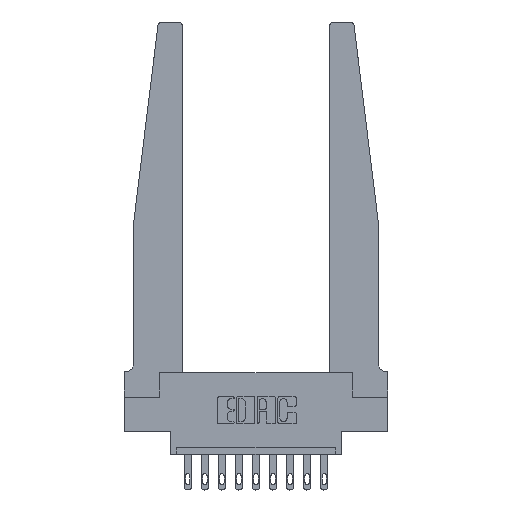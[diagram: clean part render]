
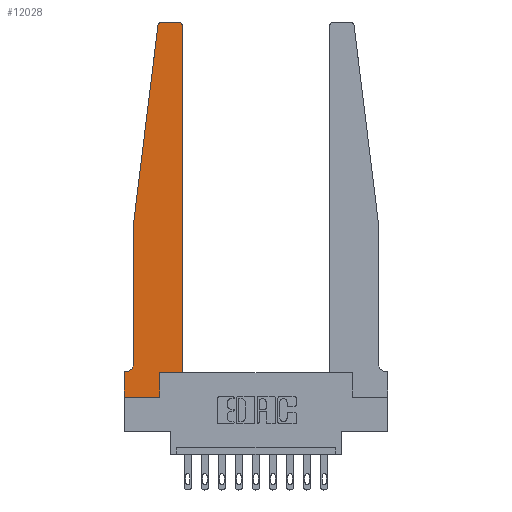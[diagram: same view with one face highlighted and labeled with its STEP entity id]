
A CAD part, top view. The second image highlights one B-rep face of the part: STEP entity #12028.
In plain terms, the highlighted planar face has unit normal (0, 0, 1).
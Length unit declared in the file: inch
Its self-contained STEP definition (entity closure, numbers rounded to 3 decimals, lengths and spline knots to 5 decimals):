
#221 = DIRECTION ( 'NONE',  ( -1., 0., 0. ) ) ;
#763 = ORIENTED_EDGE ( 'NONE', *, *, #5011, .T. ) ;
#813 = EDGE_CURVE ( 'NONE', #10666, #7998, #6678, .T. ) ;
#850 = EDGE_CURVE ( 'NONE', #5270, #13004, #12733, .T. ) ;
#868 = DIRECTION ( 'NONE',  ( 1., 0., 0. ) ) ;
#1016 = DIRECTION ( 'NONE',  ( 0., 0., 1. ) ) ;
#1043 = EDGE_CURVE ( 'NONE', #7309, #5270, #9186, .T. ) ;
#1405 = ORIENTED_EDGE ( 'NONE', *, *, #11373, .T. ) ;
#1758 = ORIENTED_EDGE ( 'NONE', *, *, #3861, .T. ) ;
#1767 = VERTEX_POINT ( 'NONE', #14062 ) ;
#2105 = DIRECTION ( 'NONE',  ( -0.122, -0.992, 0. ) ) ;
#2142 = ORIENTED_EDGE ( 'NONE', *, *, #10994, .T. ) ;
#2347 = CARTESIAN_POINT ( 'NONE',  ( 0., 0.1875, 0.37 ) ) ;
#2426 = ORIENTED_EDGE ( 'NONE', *, *, #3804, .T. ) ;
#2556 = VECTOR ( 'NONE', #3818, 39.37008 ) ;
#2643 = DIRECTION ( 'NONE',  ( -1., 0., 0. ) ) ;
#2780 = LINE ( 'NONE', #10734, #3849 ) ;
#2828 = DIRECTION ( 'NONE',  ( -1., 0., 0. ) ) ;
#2833 = AXIS2_PLACEMENT_3D ( 'NONE', #4006, #8674, #2828 ) ;
#2922 = AXIS2_PLACEMENT_3D ( 'NONE', #9887, #3920, #2981 ) ;
#2929 = VECTOR ( 'NONE', #2105, 39.37008 ) ;
#2981 = DIRECTION ( 'NONE',  ( 1., 0., 0. ) ) ;
#3204 = DIRECTION ( 'NONE',  ( 0., 1., 0. ) ) ;
#3804 = EDGE_CURVE ( 'NONE', #13603, #10203, #5160, .T. ) ;
#3818 = DIRECTION ( 'NONE',  ( 0., -1., 0. ) ) ;
#3849 = VECTOR ( 'NONE', #2643, 39.37008 ) ;
#3861 = EDGE_CURVE ( 'NONE', #6437, #1767, #8073, .T. ) ;
#3920 = DIRECTION ( 'NONE',  ( 0., 0., 1. ) ) ;
#4006 = CARTESIAN_POINT ( 'NONE',  ( 0.015, 0.2375, 0.37 ) ) ;
#4230 = ORIENTED_EDGE ( 'NONE', *, *, #12206, .T. ) ;
#4624 = CARTESIAN_POINT ( 'NONE',  ( 0.015, 0.1875, 0.37 ) ) ;
#4827 = CARTESIAN_POINT ( 'NONE',  ( 0.425, 2.72, 0.37 ) ) ;
#4849 = CARTESIAN_POINT ( 'NONE',  ( 0.065, 1.25, 0.37 ) ) ;
#4866 = DIRECTION ( 'NONE',  ( 0., 1., 0. ) ) ;
#4921 = CARTESIAN_POINT ( 'NONE',  ( 0., 0., 0.37 ) ) ;
#5011 = EDGE_CURVE ( 'NONE', #9158, #6437, #11767, .T. ) ;
#5136 = VECTOR ( 'NONE', #4866, 39.37008 ) ;
#5160 = CIRCLE ( 'NONE', #2922, 0.03 ) ;
#5270 = VERTEX_POINT ( 'NONE', #9906 ) ;
#5811 = CIRCLE ( 'NONE', #2833, 0.05 ) ;
#5851 = VERTEX_POINT ( 'NONE', #4624 ) ;
#6122 = CARTESIAN_POINT ( 'NONE',  ( 0.25, 2.75, 0.37 ) ) ;
#6144 = CARTESIAN_POINT ( 'NONE',  ( 0., 0., 0.37 ) ) ;
#6437 = VERTEX_POINT ( 'NONE', #4827 ) ;
#6678 = LINE ( 'NONE', #6756, #11085 ) ;
#6756 = CARTESIAN_POINT ( 'NONE',  ( 0.065, 1.25, 0.37 ) ) ;
#6792 = ORIENTED_EDGE ( 'NONE', *, *, #12087, .T. ) ;
#6831 = CARTESIAN_POINT ( 'NONE',  ( 0.2605, 0.18, 0.37 ) ) ;
#7046 = EDGE_LOOP ( 'NONE', ( #1405, #2426, #6792, #9996, #14518, #2142, #4230, #10807, #9471, #10648, #763, #1758 ) ) ;
#7301 = DIRECTION ( 'NONE',  ( 1., 0., 0. ) ) ;
#7309 = VERTEX_POINT ( 'NONE', #4921 ) ;
#7998 = VERTEX_POINT ( 'NONE', #11389 ) ;
#8073 = CIRCLE ( 'NONE', #15016, 0.03 ) ;
#8192 = PLANE ( 'NONE',  #9565 ) ;
#8304 = CARTESIAN_POINT ( 'NONE',  ( 0.2605, 0.18, 0.37 ) ) ;
#8449 = VECTOR ( 'NONE', #221, 39.37008 ) ;
#8674 = DIRECTION ( 'NONE',  ( 0., 0., -1. ) ) ;
#8706 = CARTESIAN_POINT ( 'NONE',  ( 0.425, 0.18, 0.37 ) ) ;
#9158 = VERTEX_POINT ( 'NONE', #8706 ) ;
#9186 = LINE ( 'NONE', #12478, #12555 ) ;
#9202 = DIRECTION ( 'NONE',  ( 0., -1., 0. ) ) ;
#9471 = ORIENTED_EDGE ( 'NONE', *, *, #850, .T. ) ;
#9565 = AXIS2_PLACEMENT_3D ( 'NONE', #2347, #1016, #11498 ) ;
#9887 = CARTESIAN_POINT ( 'NONE',  ( 0.27653, 2.72, 0.37 ) ) ;
#9906 = CARTESIAN_POINT ( 'NONE',  ( 0.2605, 0., 0.37 ) ) ;
#9996 = ORIENTED_EDGE ( 'NONE', *, *, #813, .T. ) ;
#10203 = VERTEX_POINT ( 'NONE', #12838 ) ;
#10346 = EDGE_CURVE ( 'NONE', #7998, #5851, #5811, .T. ) ;
#10500 = LINE ( 'NONE', #4849, #2929 ) ;
#10648 = ORIENTED_EDGE ( 'NONE', *, *, #12877, .T. ) ;
#10666 = VERTEX_POINT ( 'NONE', #14852 ) ;
#10727 = CARTESIAN_POINT ( 'NONE',  ( 0.27653, 2.75, 0.37 ) ) ;
#10734 = CARTESIAN_POINT ( 'NONE',  ( 0.065, 0.1875, 0.37 ) ) ;
#10807 = ORIENTED_EDGE ( 'NONE', *, *, #1043, .T. ) ;
#10994 = EDGE_CURVE ( 'NONE', #5851, #14843, #2780, .T. ) ;
#11085 = VECTOR ( 'NONE', #9202, 39.37008 ) ;
#11373 = EDGE_CURVE ( 'NONE', #1767, #13603, #14209, .T. ) ;
#11389 = CARTESIAN_POINT ( 'NONE',  ( 0.065, 0.2375, 0.37 ) ) ;
#11478 = CARTESIAN_POINT ( 'NONE',  ( 0., 0.1875, 0.37 ) ) ;
#11498 = DIRECTION ( 'NONE',  ( 1., 0., 0. ) ) ;
#11508 = DIRECTION ( 'NONE',  ( 0., 0., 1. ) ) ;
#11608 = CARTESIAN_POINT ( 'NONE',  ( 0.425, 0.18, 0.37 ) ) ;
#11767 = LINE ( 'NONE', #11608, #5136 ) ;
#12001 = LINE ( 'NONE', #14346, #13408 ) ;
#12028 = ADVANCED_FACE ( 'NONE', ( #12657 ), #8192, .T. ) ;
#12087 = EDGE_CURVE ( 'NONE', #10203, #10666, #10500, .T. ) ;
#12206 = EDGE_CURVE ( 'NONE', #14843, #7309, #13050, .T. ) ;
#12478 = CARTESIAN_POINT ( 'NONE',  ( 0., 0., 0.37 ) ) ;
#12551 = DIRECTION ( 'NONE',  ( 1., 0., 0. ) ) ;
#12555 = VECTOR ( 'NONE', #12551, 39.37008 ) ;
#12657 = FACE_OUTER_BOUND ( 'NONE', #7046, .T. ) ;
#12733 = LINE ( 'NONE', #6831, #14317 ) ;
#12838 = CARTESIAN_POINT ( 'NONE',  ( 0.24675, 2.72367, 0.37 ) ) ;
#12877 = EDGE_CURVE ( 'NONE', #13004, #9158, #12001, .T. ) ;
#13004 = VERTEX_POINT ( 'NONE', #8304 ) ;
#13050 = LINE ( 'NONE', #6144, #2556 ) ;
#13408 = VECTOR ( 'NONE', #7301, 39.37008 ) ;
#13603 = VERTEX_POINT ( 'NONE', #10727 ) ;
#13620 = CARTESIAN_POINT ( 'NONE',  ( 0.395, 2.72, 0.37 ) ) ;
#14062 = CARTESIAN_POINT ( 'NONE',  ( 0.395, 2.75, 0.37 ) ) ;
#14209 = LINE ( 'NONE', #6122, #8449 ) ;
#14317 = VECTOR ( 'NONE', #3204, 39.37008 ) ;
#14346 = CARTESIAN_POINT ( 'NONE',  ( 0.425, 0.18, 0.37 ) ) ;
#14518 = ORIENTED_EDGE ( 'NONE', *, *, #10346, .T. ) ;
#14843 = VERTEX_POINT ( 'NONE', #11478 ) ;
#14852 = CARTESIAN_POINT ( 'NONE',  ( 0.065, 1.25, 0.37 ) ) ;
#15016 = AXIS2_PLACEMENT_3D ( 'NONE', #13620, #11508, #868 ) ;
